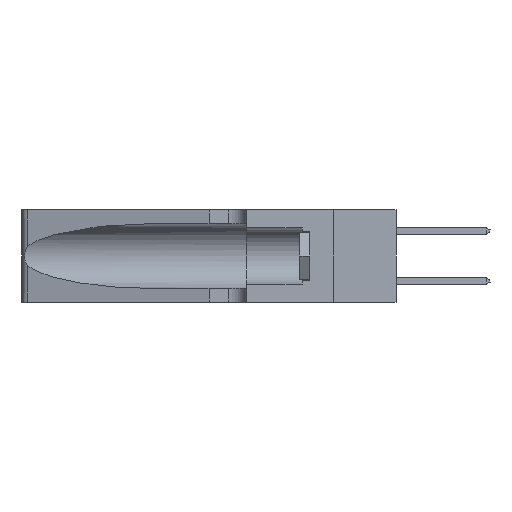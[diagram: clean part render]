
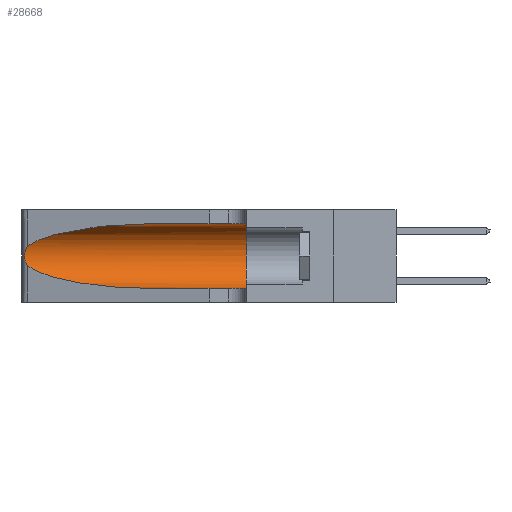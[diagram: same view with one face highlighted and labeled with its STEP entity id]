
A CAD part, left-side view. The second image highlights one B-rep face of the part: STEP entity #28668.
In plain terms, the highlighted cylindrical face has radius 3.308 mm (diameter 6.617 mm), a partial arc.
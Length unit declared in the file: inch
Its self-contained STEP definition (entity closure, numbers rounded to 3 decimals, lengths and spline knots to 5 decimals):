
#239 = ORIENTED_EDGE ( 'NONE', *, *, #26451, .T. ) ;
#656 = CARTESIAN_POINT ( 'NONE',  ( 0.1305, 1.61858, 0.185 ) ) ;
#973 = FACE_OUTER_BOUND ( 'NONE', #16256, .T. ) ;
#1855 = CARTESIAN_POINT ( 'NONE',  ( 0.18966, 0.96281, 0.31525 ) ) ;
#2006 =( BOUNDED_CURVE ( )  B_SPLINE_CURVE ( 3, ( #12631, #1855, #28600, #12748 ),
 .UNSPECIFIED., .F., .F. ) 
 B_SPLINE_CURVE_WITH_KNOTS ( ( 4, 4 ),
 ( 1.5708, 2.84003 ),
 .UNSPECIFIED. ) 
 CURVE ( )  GEOMETRIC_REPRESENTATION_ITEM ( )  RATIONAL_B_SPLINE_CURVE ( ( 1., 0.87, 0.87, 1. ) ) 
 REPRESENTATION_ITEM ( '' )  );
#2106 = CARTESIAN_POINT ( 'NONE',  ( 0.26018, 1.23835, 0.19895 ) ) ;
#3057 = ORIENTED_EDGE ( 'NONE', *, *, #23277, .F. ) ;
#3286 = EDGE_CURVE ( 'NONE', #29987, #8606, #32933, .T. ) ;
#4563 = LINE ( 'NONE', #16120, #18042 ) ;
#4820 = CARTESIAN_POINT ( 'NONE',  ( 0.26075, 1.23896, 0.178 ) ) ;
#4989 = CARTESIAN_POINT ( 'NONE',  ( 0.25487, 1.22718, 0.22369 ) ) ;
#5317 = VERTEX_POINT ( 'NONE', #19036 ) ;
#7328 = ORIENTED_EDGE ( 'NONE', *, *, #32556, .F. ) ;
#7535 = CARTESIAN_POINT ( 'NONE',  ( 0.25856, 1.23593, 0.16098 ) ) ;
#8606 = VERTEX_POINT ( 'NONE', #15858 ) ;
#9575 = VERTEX_POINT ( 'NONE', #24729 ) ;
#10178 = CARTESIAN_POINT ( 'NONE',  ( 0.25639, 1.23184, 0.21858 ) ) ;
#10301 = CARTESIAN_POINT ( 'NONE',  ( 0.25639, 1.23186, 0.15144 ) ) ;
#11068 = CARTESIAN_POINT ( 'NONE',  ( 0.1305, 0.35, 0.31525 ) ) ;
#11578 = DIRECTION ( 'NONE',  ( 0., -1., 0. ) ) ;
#12631 = CARTESIAN_POINT ( 'NONE',  ( 0.1305, 0.72297, 0.31525 ) ) ;
#12748 = CARTESIAN_POINT ( 'NONE',  ( 0.25487, 1.22718, 0.22369 ) ) ;
#12862 = CARTESIAN_POINT ( 'NONE',  ( 0.2373, 1.15595, 0.08982 ) ) ;
#12976 = CARTESIAN_POINT ( 'NONE',  ( 0.1305, 0.72297, 0.05475 ) ) ;
#12982 = CARTESIAN_POINT ( 'NONE',  ( 0.25487, 1.22718, 0.14631 ) ) ;
#13323 = VERTEX_POINT ( 'NONE', #18082 ) ;
#13619 = VERTEX_POINT ( 'NONE', #11068 ) ;
#14498 = CYLINDRICAL_SURFACE ( 'NONE', #31876, 0.13025 ) ;
#14666 = DIRECTION ( 'NONE',  ( 0., 1., 0. ) ) ;
#15551 = CARTESIAN_POINT ( 'NONE',  ( 0.25487, 1.22718, 0.22369 ) ) ;
#15858 = CARTESIAN_POINT ( 'NONE',  ( 0.25487, 1.22718, 0.14631 ) ) ;
#16120 = CARTESIAN_POINT ( 'NONE',  ( 0.1305, 1.61858, 0.31525 ) ) ;
#16256 = EDGE_LOOP ( 'NONE', ( #30042, #22128, #239, #33878, #3057, #7328 ) ) ;
#16834 = DIRECTION ( 'NONE',  ( 0., 0., -1. ) ) ;
#18042 = VECTOR ( 'NONE', #18815, 39.37008 ) ;
#18082 = CARTESIAN_POINT ( 'NONE',  ( 0.1305, 0.72297, 0.05475 ) ) ;
#18250 = CARTESIAN_POINT ( 'NONE',  ( 0.25854, 1.2359, 0.20912 ) ) ;
#18815 = DIRECTION ( 'NONE',  ( 0., -1., 0. ) ) ;
#19036 = CARTESIAN_POINT ( 'NONE',  ( 0.1305, 0.35, 0.05475 ) ) ;
#20559 = VECTOR ( 'NONE', #31765, 39.37008 ) ;
#20936 = CARTESIAN_POINT ( 'NONE',  ( 0.26075, 1.23896, 0.19203 ) ) ;
#21269 = CIRCLE ( 'NONE', #25379, 0.13025 ) ;
#22128 = ORIENTED_EDGE ( 'NONE', *, *, #3286, .T. ) ;
#23277 = EDGE_CURVE ( 'NONE', #13619, #5317, #21269, .T. ) ;
#23554 = CARTESIAN_POINT ( 'NONE',  ( 0.25487, 1.22718, 0.14631 ) ) ;
#23559 = CARTESIAN_POINT ( 'NONE',  ( 0.26017, 1.23833, 0.17102 ) ) ;
#24358 =( BOUNDED_CURVE ( )  B_SPLINE_CURVE ( 3, ( #23554, #12862, #28814, #12976 ),
 .UNSPECIFIED., .F., .F. ) 
 B_SPLINE_CURVE_WITH_KNOTS ( ( 4, 4 ),
 ( 3.44316, 4.71239 ),
 .UNSPECIFIED. ) 
 CURVE ( )  GEOMETRIC_REPRESENTATION_ITEM ( )  RATIONAL_B_SPLINE_CURVE ( ( 1., 0.87, 0.87, 1. ) ) 
 REPRESENTATION_ITEM ( '' )  );
#24612 = EDGE_CURVE ( 'NONE', #9575, #29987, #2006, .T. ) ;
#24729 = CARTESIAN_POINT ( 'NONE',  ( 0.1305, 0.72297, 0.31525 ) ) ;
#25379 = AXIS2_PLACEMENT_3D ( 'NONE', #30467, #14666, #33082 ) ;
#26199 = CARTESIAN_POINT ( 'NONE',  ( 0.25789, 1.23486, 0.15765 ) ) ;
#26451 = EDGE_CURVE ( 'NONE', #8606, #13323, #24358, .T. ) ;
#27516 = LINE ( 'NONE', #29146, #20559 ) ;
#28600 = CARTESIAN_POINT ( 'NONE',  ( 0.2373, 1.15595, 0.28018 ) ) ;
#28668 = ADVANCED_FACE ( 'NONE', ( #973 ), #14498, .F. ) ;
#28717 = CARTESIAN_POINT ( 'NONE',  ( 0.25555, 1.22994, 0.2215 ) ) ;
#28814 = CARTESIAN_POINT ( 'NONE',  ( 0.18966, 0.96281, 0.05475 ) ) ;
#28821 = CARTESIAN_POINT ( 'NONE',  ( 0.25555, 1.22993, 0.14849 ) ) ;
#29146 = CARTESIAN_POINT ( 'NONE',  ( 0.1305, 1.61858, 0.05475 ) ) ;
#29987 = VERTEX_POINT ( 'NONE', #4989 ) ;
#30042 = ORIENTED_EDGE ( 'NONE', *, *, #24612, .T. ) ;
#30467 = CARTESIAN_POINT ( 'NONE',  ( 0.1305, 0.35, 0.185 ) ) ;
#31765 = DIRECTION ( 'NONE',  ( 0., -1., 0. ) ) ;
#31876 = AXIS2_PLACEMENT_3D ( 'NONE', #656, #11578, #16834 ) ;
#32501 = EDGE_CURVE ( 'NONE', #13323, #5317, #27516, .T. ) ;
#32556 = EDGE_CURVE ( 'NONE', #9575, #13619, #4563, .T. ) ;
#32933 = B_SPLINE_CURVE_WITH_KNOTS ( 'NONE', 3,
 ( #15551, #28717, #10178, #33944, #18250, #2106, #20936, #4820, #23559, #7535, #26199, #10301, #28821, #12982 ),
 .UNSPECIFIED., .F., .F.,
 ( 4, 2, 2, 2, 2, 2, 4 ),
 ( 0., 0.00027, 0.00053, 0.00107, 0.0016, 0.00187, 0.00214 ),
 .UNSPECIFIED. ) ;
#33082 = DIRECTION ( 'NONE',  ( 0., 0., 1. ) ) ;
#33878 = ORIENTED_EDGE ( 'NONE', *, *, #32501, .T. ) ;
#33944 = CARTESIAN_POINT ( 'NONE',  ( 0.25787, 1.23484, 0.2124 ) ) ;
